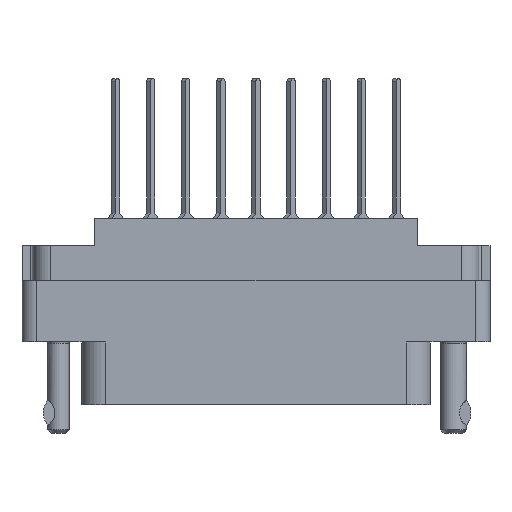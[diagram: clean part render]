
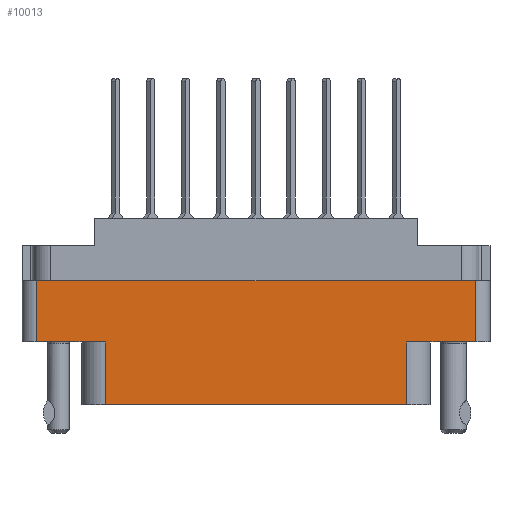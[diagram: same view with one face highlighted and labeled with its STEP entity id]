
A CAD part, front view. The second image highlights one B-rep face of the part: STEP entity #10013.
In plain terms, the highlighted planar face has unit normal (0, -1, 0).
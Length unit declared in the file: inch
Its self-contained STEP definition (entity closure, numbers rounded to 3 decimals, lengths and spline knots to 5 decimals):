
#78 = VERTEX_POINT ( 'NONE', #42981 ) ;
#606 = CARTESIAN_POINT ( 'NONE',  ( 0.938, -0.438, -0.798 ) ) ;
#1122 = VERTEX_POINT ( 'NONE', #7458 ) ;
#1197 = CARTESIAN_POINT ( 'NONE',  ( -1., -0.438, -0.268 ) ) ;
#2411 = LINE ( 'NONE', #19062, #11816 ) ;
#3281 = CARTESIAN_POINT ( 'NONE',  ( -0.644, -0.438, -0.798 ) ) ;
#3615 = EDGE_CURVE ( 'NONE', #9496, #32668, #15503, .T. ) ;
#5495 = CARTESIAN_POINT ( 'NONE',  ( 0.938, -0.438, -0.268 ) ) ;
#6960 = ORIENTED_EDGE ( 'NONE', *, *, #28966, .T. ) ;
#7394 = EDGE_CURVE ( 'NONE', #1122, #33498, #27005, .T. ) ;
#7458 = CARTESIAN_POINT ( 'NONE',  ( 0.644, -0.438, -0.529 ) ) ;
#7718 = LINE ( 'NONE', #18279, #41479 ) ;
#9496 = VERTEX_POINT ( 'NONE', #13296 ) ;
#9695 = DIRECTION ( 'NONE',  ( 0., 0., -1. ) ) ;
#10013 = ADVANCED_FACE ( 'NONE', ( #37328 ), #28985, .T. ) ;
#10460 = VECTOR ( 'NONE', #9695, 39.37008 ) ;
#11426 = DIRECTION ( 'NONE',  ( 0., 0., 1. ) ) ;
#11710 = CARTESIAN_POINT ( 'NONE',  ( -0.938, -0.438, -0.798 ) ) ;
#11816 = VECTOR ( 'NONE', #19218, 39.37008 ) ;
#13296 = CARTESIAN_POINT ( 'NONE',  ( -0.938, -0.438, -0.529 ) ) ;
#14797 = VERTEX_POINT ( 'NONE', #31119 ) ;
#15071 = CARTESIAN_POINT ( 'NONE',  ( 0.644, -0.438, -0.798 ) ) ;
#15503 = LINE ( 'NONE', #22120, #38793 ) ;
#16050 = EDGE_LOOP ( 'NONE', ( #35544, #21738, #29464, #30501, #6960, #22067, #41421, #45662 ) ) ;
#16130 = VECTOR ( 'NONE', #40738, 39.37008 ) ;
#18128 = DIRECTION ( 'NONE',  ( -1., 0., 0. ) ) ;
#18279 = CARTESIAN_POINT ( 'NONE',  ( 0., -0.438, -0.529 ) ) ;
#18453 = LINE ( 'NONE', #1197, #24549 ) ;
#18696 = VECTOR ( 'NONE', #27685, 39.37008 ) ;
#19062 = CARTESIAN_POINT ( 'NONE',  ( 0., -0.438, -0.529 ) ) ;
#19218 = DIRECTION ( 'NONE',  ( 1., 0., 0. ) ) ;
#21738 = ORIENTED_EDGE ( 'NONE', *, *, #44331, .T. ) ;
#22067 = ORIENTED_EDGE ( 'NONE', *, *, #25379, .F. ) ;
#22120 = CARTESIAN_POINT ( 'NONE',  ( -0.938, -0.438, -0.798 ) ) ;
#22903 = CARTESIAN_POINT ( 'NONE',  ( -0.938, -0.438, -0.798 ) ) ;
#23115 = VECTOR ( 'NONE', #11426, 39.37008 ) ;
#23861 = VERTEX_POINT ( 'NONE', #5495 ) ;
#23917 = AXIS2_PLACEMENT_3D ( 'NONE', #11710, #39833, #25577 ) ;
#24549 = VECTOR ( 'NONE', #29302, 39.37008 ) ;
#25333 = CARTESIAN_POINT ( 'NONE',  ( -0.938, -0.438, -0.268 ) ) ;
#25379 = EDGE_CURVE ( 'NONE', #32668, #23861, #18453, .T. ) ;
#25518 = EDGE_CURVE ( 'NONE', #9496, #14797, #2411, .T. ) ;
#25577 = DIRECTION ( 'NONE',  ( 0., 0., -1. ) ) ;
#26448 = LINE ( 'NONE', #606, #23115 ) ;
#27005 = LINE ( 'NONE', #30719, #10460 ) ;
#27685 = DIRECTION ( 'NONE',  ( 0., 0., -1. ) ) ;
#28966 = EDGE_CURVE ( 'NONE', #78, #23861, #26448, .T. ) ;
#28985 = PLANE ( 'NONE',  #23917 ) ;
#29233 = LINE ( 'NONE', #42076, #18696 ) ;
#29302 = DIRECTION ( 'NONE',  ( 1., 0., 0. ) ) ;
#29464 = ORIENTED_EDGE ( 'NONE', *, *, #7394, .F. ) ;
#29744 = DIRECTION ( 'NONE',  ( 0., 0., 1. ) ) ;
#30501 = ORIENTED_EDGE ( 'NONE', *, *, #39543, .F. ) ;
#30719 = CARTESIAN_POINT ( 'NONE',  ( 0.644, -0.438, -0.529 ) ) ;
#31119 = CARTESIAN_POINT ( 'NONE',  ( -0.644, -0.438, -0.529 ) ) ;
#32431 = EDGE_CURVE ( 'NONE', #14797, #43433, #29233, .T. ) ;
#32668 = VERTEX_POINT ( 'NONE', #25333 ) ;
#33498 = VERTEX_POINT ( 'NONE', #15071 ) ;
#35544 = ORIENTED_EDGE ( 'NONE', *, *, #32431, .T. ) ;
#37193 = LINE ( 'NONE', #22903, #16130 ) ;
#37328 = FACE_OUTER_BOUND ( 'NONE', #16050, .T. ) ;
#38793 = VECTOR ( 'NONE', #29744, 39.37008 ) ;
#39543 = EDGE_CURVE ( 'NONE', #78, #1122, #7718, .T. ) ;
#39833 = DIRECTION ( 'NONE',  ( 0., -1., 0. ) ) ;
#40738 = DIRECTION ( 'NONE',  ( 1., 0., 0. ) ) ;
#41421 = ORIENTED_EDGE ( 'NONE', *, *, #3615, .F. ) ;
#41479 = VECTOR ( 'NONE', #18128, 39.37008 ) ;
#42076 = CARTESIAN_POINT ( 'NONE',  ( -0.644, -0.438, -0.529 ) ) ;
#42981 = CARTESIAN_POINT ( 'NONE',  ( 0.938, -0.438, -0.529 ) ) ;
#43433 = VERTEX_POINT ( 'NONE', #3281 ) ;
#44331 = EDGE_CURVE ( 'NONE', #43433, #33498, #37193, .T. ) ;
#45662 = ORIENTED_EDGE ( 'NONE', *, *, #25518, .T. ) ;
